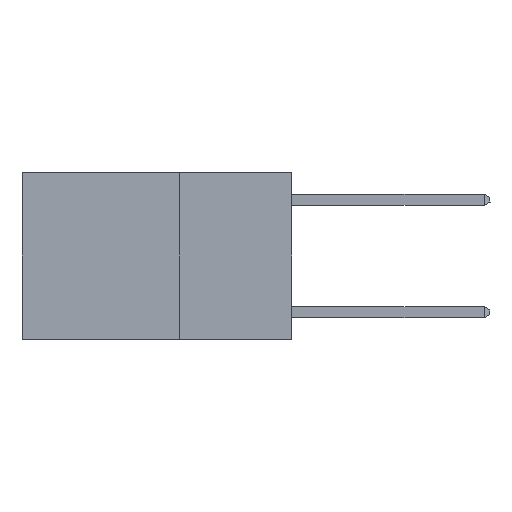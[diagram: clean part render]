
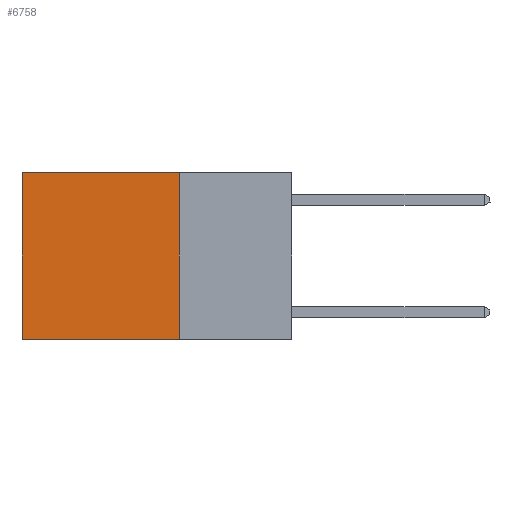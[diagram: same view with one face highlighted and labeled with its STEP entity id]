
A CAD part, left-side view. The second image highlights one B-rep face of the part: STEP entity #6758.
In plain terms, the highlighted planar face has unit normal (-1, 0, 0).
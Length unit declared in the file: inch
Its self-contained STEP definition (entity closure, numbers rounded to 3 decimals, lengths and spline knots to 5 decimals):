
#100 = CARTESIAN_POINT ( 'NONE',  ( 0.2625, 0.6, 0. ) ) ;
#303 = DIRECTION ( 'NONE',  ( 0., 0., -1. ) ) ;
#465 = ORIENTED_EDGE ( 'NONE', *, *, #11948, .F. ) ;
#674 = DIRECTION ( 'NONE',  ( 0., 1., 0. ) ) ;
#713 = CARTESIAN_POINT ( 'NONE',  ( 0.2625, 0.25, -0.37 ) ) ;
#1122 = VECTOR ( 'NONE', #8846, 39.37008 ) ;
#1193 = FACE_OUTER_BOUND ( 'NONE', #10238, .T. ) ;
#1219 = DIRECTION ( 'NONE',  ( 0., 0., -1. ) ) ;
#2317 = CARTESIAN_POINT ( 'NONE',  ( 0.2625, 0.25, 0. ) ) ;
#2345 = VERTEX_POINT ( 'NONE', #713 ) ;
#2545 = ORIENTED_EDGE ( 'NONE', *, *, #8881, .T. ) ;
#2615 = VECTOR ( 'NONE', #1219, 39.37008 ) ;
#2629 = VERTEX_POINT ( 'NONE', #100 ) ;
#4254 = EDGE_CURVE ( 'NONE', #9998, #2629, #8206, .T. ) ;
#4632 = ORIENTED_EDGE ( 'NONE', *, *, #4254, .T. ) ;
#5961 = CARTESIAN_POINT ( 'NONE',  ( 0.2625, 0.25, 0. ) ) ;
#6758 = ADVANCED_FACE ( 'NONE', ( #1193 ), #8511, .F. ) ;
#7214 = CARTESIAN_POINT ( 'NONE',  ( 0.2625, 0.6, -0.37 ) ) ;
#7930 = LINE ( 'NONE', #13458, #8096 ) ;
#8096 = VECTOR ( 'NONE', #303, 39.37008 ) ;
#8206 = LINE ( 'NONE', #8838, #8529 ) ;
#8511 = PLANE ( 'NONE',  #11073 ) ;
#8529 = VECTOR ( 'NONE', #674, 39.37008 ) ;
#8776 = LINE ( 'NONE', #9668, #2615 ) ;
#8838 = CARTESIAN_POINT ( 'NONE',  ( 0.2625, 0.25, 0. ) ) ;
#8846 = DIRECTION ( 'NONE',  ( 0., 1., 0. ) ) ;
#8854 = VERTEX_POINT ( 'NONE', #7214 ) ;
#8881 = EDGE_CURVE ( 'NONE', #2629, #8854, #7930, .T. ) ;
#8967 = EDGE_CURVE ( 'NONE', #2345, #8854, #12486, .T. ) ;
#9588 = DIRECTION ( 'NONE',  ( 0., 0., -1. ) ) ;
#9668 = CARTESIAN_POINT ( 'NONE',  ( 0.2625, 0.25, 0. ) ) ;
#9998 = VERTEX_POINT ( 'NONE', #5961 ) ;
#10238 = EDGE_LOOP ( 'NONE', ( #2545, #10610, #465, #4632 ) ) ;
#10610 = ORIENTED_EDGE ( 'NONE', *, *, #8967, .F. ) ;
#10675 = DIRECTION ( 'NONE',  ( 1., 0., 0. ) ) ;
#11073 = AXIS2_PLACEMENT_3D ( 'NONE', #2317, #10675, #9588 ) ;
#11948 = EDGE_CURVE ( 'NONE', #9998, #2345, #8776, .T. ) ;
#12486 = LINE ( 'NONE', #12706, #1122 ) ;
#12706 = CARTESIAN_POINT ( 'NONE',  ( 0.2625, 0.25, -0.37 ) ) ;
#13458 = CARTESIAN_POINT ( 'NONE',  ( 0.2625, 0.6, 0. ) ) ;
